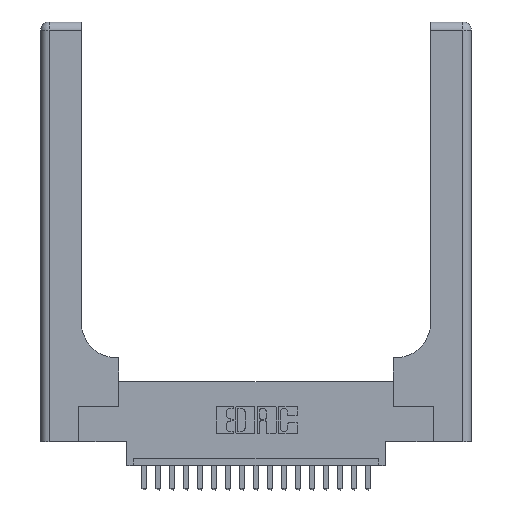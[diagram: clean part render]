
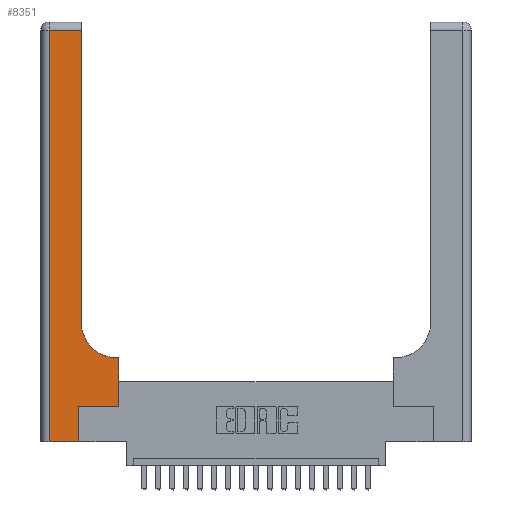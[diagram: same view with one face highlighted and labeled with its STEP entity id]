
A CAD part, top view. The second image highlights one B-rep face of the part: STEP entity #8351.
In plain terms, the highlighted planar face has unit normal (0, 0, 1).
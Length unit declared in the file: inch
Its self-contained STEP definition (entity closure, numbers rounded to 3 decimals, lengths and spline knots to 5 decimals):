
#1 = CARTESIAN_POINT ( 'NONE',  ( 0.5585, 0.25, 0.37 ) ) ;
#7 = CARTESIAN_POINT ( 'NONE',  ( 0.5415, 0.85, 0.37 ) ) ;
#279 = CARTESIAN_POINT ( 'NONE',  ( 0.269, 0.25, 0.37 ) ) ;
#310 = DIRECTION ( 'NONE',  ( 0., 0., -1. ) ) ;
#475 = VERTEX_POINT ( 'NONE', #15182 ) ;
#582 = VECTOR ( 'NONE', #15440, 39.37008 ) ;
#724 = CARTESIAN_POINT ( 'NONE',  ( 0.06, 0., 0.37 ) ) ;
#1185 = CARTESIAN_POINT ( 'NONE',  ( 0.5415, 0.6, 0.37 ) ) ;
#1288 = LINE ( 'NONE', #3022, #1824 ) ;
#1824 = VECTOR ( 'NONE', #16329, 39.37008 ) ;
#1965 = EDGE_CURVE ( 'NONE', #475, #4843, #18625, .T. ) ;
#2586 = DIRECTION ( 'NONE',  ( 0., 0., -1. ) ) ;
#2976 = VERTEX_POINT ( 'NONE', #5393 ) ;
#3006 = ORIENTED_EDGE ( 'NONE', *, *, #16378, .T. ) ;
#3022 = CARTESIAN_POINT ( 'NONE',  ( 0.06, 3., 0.37 ) ) ;
#3342 = DIRECTION ( 'NONE',  ( 0., 1., 0. ) ) ;
#3485 = DIRECTION ( 'NONE',  ( 1., 0., 0. ) ) ;
#3700 = VECTOR ( 'NONE', #16749, 39.37008 ) ;
#3803 = EDGE_CURVE ( 'NONE', #19986, #9970, #15966, .T. ) ;
#3857 = ORIENTED_EDGE ( 'NONE', *, *, #16235, .T. ) ;
#4341 = ORIENTED_EDGE ( 'NONE', *, *, #8160, .T. ) ;
#4843 = VERTEX_POINT ( 'NONE', #11879 ) ;
#4977 = LINE ( 'NONE', #14983, #3700 ) ;
#5393 = CARTESIAN_POINT ( 'NONE',  ( 0.2915, 0.85, 0.37 ) ) ;
#5994 = EDGE_CURVE ( 'NONE', #2976, #475, #4977, .T. ) ;
#6661 = CARTESIAN_POINT ( 'NONE',  ( 0.269, 0., 0.37 ) ) ;
#6949 = PLANE ( 'NONE',  #15597 ) ;
#7389 = EDGE_CURVE ( 'NONE', #16843, #9682, #14497, .T. ) ;
#7534 = DIRECTION ( 'NONE',  ( -1., 0., 0. ) ) ;
#7559 = EDGE_LOOP ( 'NONE', ( #15612, #13992, #18743, #13712, #4341, #15270, #3006, #18710, #3857 ) ) ;
#7668 = LINE ( 'NONE', #17153, #14144 ) ;
#8160 = EDGE_CURVE ( 'NONE', #9682, #19986, #19973, .T. ) ;
#8248 = FACE_OUTER_BOUND ( 'NONE', #7559, .T. ) ;
#8351 = ADVANCED_FACE ( 'NONE', ( #8248 ), #6949, .F. ) ;
#8734 = VERTEX_POINT ( 'NONE', #18266 ) ;
#8756 = CARTESIAN_POINT ( 'NONE',  ( 0.2915, 0.6, 0.37 ) ) ;
#9682 = VERTEX_POINT ( 'NONE', #12515 ) ;
#9970 = VERTEX_POINT ( 'NONE', #1 ) ;
#9975 = CIRCLE ( 'NONE', #18287, 0.25 ) ;
#10179 = EDGE_CURVE ( 'NONE', #8734, #13226, #11748, .T. ) ;
#10256 = VECTOR ( 'NONE', #16268, 39.37008 ) ;
#10399 = DIRECTION ( 'NONE',  ( 0., 1., 0. ) ) ;
#10854 = VECTOR ( 'NONE', #3485, 39.37008 ) ;
#11748 = LINE ( 'NONE', #8756, #582 ) ;
#11784 = DIRECTION ( 'NONE',  ( 1., 0., 0. ) ) ;
#11879 = CARTESIAN_POINT ( 'NONE',  ( 0.06, 2.94, 0.37 ) ) ;
#12275 = EDGE_CURVE ( 'NONE', #4843, #16843, #1288, .T. ) ;
#12515 = CARTESIAN_POINT ( 'NONE',  ( 0.269, 0., 0.37 ) ) ;
#13226 = VERTEX_POINT ( 'NONE', #1185 ) ;
#13712 = ORIENTED_EDGE ( 'NONE', *, *, #7389, .T. ) ;
#13992 = ORIENTED_EDGE ( 'NONE', *, *, #1965, .T. ) ;
#14144 = VECTOR ( 'NONE', #10399, 39.37008 ) ;
#14497 = LINE ( 'NONE', #20201, #10854 ) ;
#14569 = CARTESIAN_POINT ( 'NONE',  ( 0., 2.94, 0.37 ) ) ;
#14983 = CARTESIAN_POINT ( 'NONE',  ( 0.2915, 3., 0.37 ) ) ;
#15182 = CARTESIAN_POINT ( 'NONE',  ( 0.2915, 2.94, 0.37 ) ) ;
#15270 = ORIENTED_EDGE ( 'NONE', *, *, #3803, .T. ) ;
#15440 = DIRECTION ( 'NONE',  ( -1., 0., 0. ) ) ;
#15597 = AXIS2_PLACEMENT_3D ( 'NONE', #18591, #2586, #7534 ) ;
#15612 = ORIENTED_EDGE ( 'NONE', *, *, #5994, .T. ) ;
#15966 = LINE ( 'NONE', #18483, #20914 ) ;
#16235 = EDGE_CURVE ( 'NONE', #13226, #2976, #9975, .T. ) ;
#16268 = DIRECTION ( 'NONE',  ( -1., 0., 0. ) ) ;
#16329 = DIRECTION ( 'NONE',  ( 0., -1., 0. ) ) ;
#16378 = EDGE_CURVE ( 'NONE', #9970, #8734, #7668, .T. ) ;
#16749 = DIRECTION ( 'NONE',  ( 0., 1., 0. ) ) ;
#16843 = VERTEX_POINT ( 'NONE', #724 ) ;
#17153 = CARTESIAN_POINT ( 'NONE',  ( 0.5585, 0.25, 0.37 ) ) ;
#18266 = CARTESIAN_POINT ( 'NONE',  ( 0.5585, 0.6, 0.37 ) ) ;
#18287 = AXIS2_PLACEMENT_3D ( 'NONE', #7, #310, #11784 ) ;
#18411 = VECTOR ( 'NONE', #3342, 39.37008 ) ;
#18483 = CARTESIAN_POINT ( 'NONE',  ( 0.269, 0.25, 0.37 ) ) ;
#18554 = DIRECTION ( 'NONE',  ( 1., 0., 0. ) ) ;
#18591 = CARTESIAN_POINT ( 'NONE',  ( 0., 3., 0.37 ) ) ;
#18625 = LINE ( 'NONE', #14569, #10256 ) ;
#18710 = ORIENTED_EDGE ( 'NONE', *, *, #10179, .T. ) ;
#18743 = ORIENTED_EDGE ( 'NONE', *, *, #12275, .T. ) ;
#19973 = LINE ( 'NONE', #6661, #18411 ) ;
#19986 = VERTEX_POINT ( 'NONE', #279 ) ;
#20201 = CARTESIAN_POINT ( 'NONE',  ( 0., 0., 0.37 ) ) ;
#20914 = VECTOR ( 'NONE', #18554, 39.37008 ) ;
